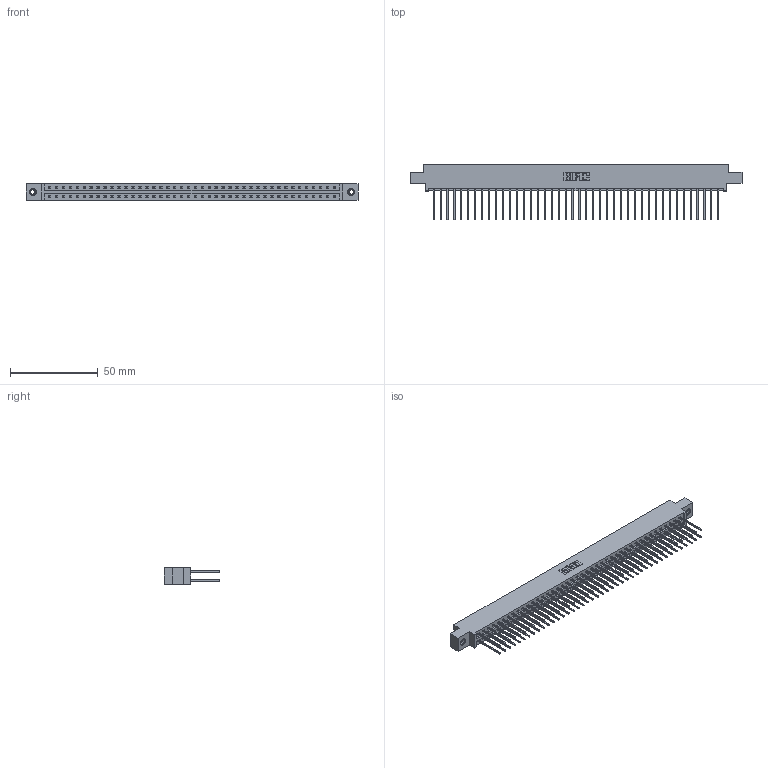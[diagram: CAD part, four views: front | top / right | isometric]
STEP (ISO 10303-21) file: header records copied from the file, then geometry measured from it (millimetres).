
FILE_DESCRIPTION (( 'STEP AP203' ), '1' );
FILE_NAME ('337-084-542-807.STEP', '2018-08-12T22:58:08', ( '' ), ( '' ), 'SwSTEP 2.0', 'SolidWorks 2016', '' );
FILE_SCHEMA (( 'CONFIG_CONTROL_DESIGN' ));
Length unit declared in the file: inch
Products named in the file (4): 337 Part_0.170 Offset - 0.156 Dia-TI; 345-292-001_345-293-142; 345-250-001_345-250-005-103; 337-084-542-807
Assembly tree (87 placements, depth 2):
  337-084-542-807
    337 Part_0.170 Offset - 0.156 Dia-TI
    345-292-001_345-293-142  x84
    345-250-001_345-250-005-103  x2
Bounding box: 189.43 x 31.63 x 9.4 mm (x, y, z)
Volume: 20224.5 mm3; surface area: 24959.8 mm2
Topology: 87 solids, 87 shells, 4714 faces, 13983 edges, 9202 vertices
Faces by surface type: plane 3298, cylinder 1400, cone 12, torus 4
Entity records: 33900 total; most frequent: CARTESIAN_POINT 5693, ORIENTED_EDGE 5622, DIRECTION 4873, EDGE_CURVE 2811, VECTOR 2663, LINE 2663, VERTEX_POINT 1868, AXIS2_PLACEMENT_3D 1105
